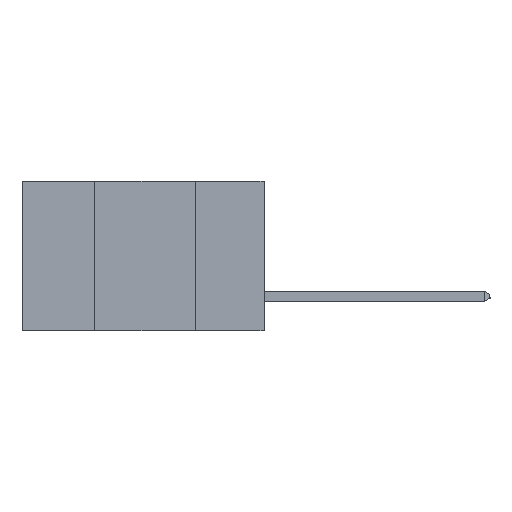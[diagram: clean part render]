
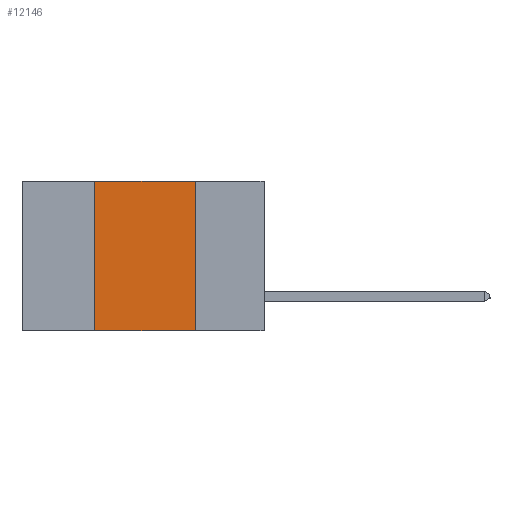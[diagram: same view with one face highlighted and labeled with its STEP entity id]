
A CAD part, left-side view. The second image highlights one B-rep face of the part: STEP entity #12146.
In plain terms, the highlighted planar face has unit normal (-1, 0, 0).
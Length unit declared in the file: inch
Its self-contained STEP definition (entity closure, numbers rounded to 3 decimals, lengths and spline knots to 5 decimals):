
#48 = FACE_OUTER_BOUND ( 'NONE', #1175, .T. ) ;
#1175 = EDGE_LOOP ( 'NONE', ( #3247, #3525, #3396, #16565 ) ) ;
#1203 = PLANE ( 'NONE',  #12071 ) ;
#1386 = VECTOR ( 'NONE', #14968, 39.37008 ) ;
#3179 = LINE ( 'NONE', #13834, #10072 ) ;
#3247 = ORIENTED_EDGE ( 'NONE', *, *, #11730, .F. ) ;
#3396 = ORIENTED_EDGE ( 'NONE', *, *, #7034, .F. ) ;
#3525 = ORIENTED_EDGE ( 'NONE', *, *, #16155, .F. ) ;
#4145 = CARTESIAN_POINT ( 'NONE',  ( 0., 0.42, 0. ) ) ;
#4399 = VECTOR ( 'NONE', #13385, 39.37008 ) ;
#4915 = VERTEX_POINT ( 'NONE', #10560 ) ;
#5005 = LINE ( 'NONE', #8406, #1386 ) ;
#7034 = EDGE_CURVE ( 'NONE', #9112, #10293, #8111, .T. ) ;
#8111 = LINE ( 'NONE', #4145, #4399 ) ;
#8406 = CARTESIAN_POINT ( 'NONE',  ( 0., 0.6, -0.37 ) ) ;
#9112 = VERTEX_POINT ( 'NONE', #11243 ) ;
#9827 = DIRECTION ( 'NONE',  ( 0., 0., -1. ) ) ;
#10072 = VECTOR ( 'NONE', #9827, 39.37008 ) ;
#10293 = VERTEX_POINT ( 'NONE', #15085 ) ;
#10560 = CARTESIAN_POINT ( 'NONE',  ( 0., 0.17, -0.37 ) ) ;
#10762 = DIRECTION ( 'NONE',  ( 0., 0., -1. ) ) ;
#10831 = CARTESIAN_POINT ( 'NONE',  ( 0., 0.6, 0. ) ) ;
#11243 = CARTESIAN_POINT ( 'NONE',  ( 0., 0.42, -0.37 ) ) ;
#11601 = VERTEX_POINT ( 'NONE', #12324 ) ;
#11730 = EDGE_CURVE ( 'NONE', #11601, #4915, #3179, .T. ) ;
#12071 = AXIS2_PLACEMENT_3D ( 'NONE', #17161, #14631, #10762 ) ;
#12146 = ADVANCED_FACE ( 'NONE', ( #48 ), #1203, .F. ) ;
#12324 = CARTESIAN_POINT ( 'NONE',  ( 0., 0.17, 0. ) ) ;
#13385 = DIRECTION ( 'NONE',  ( 0., 0., 1. ) ) ;
#13833 = LINE ( 'NONE', #10831, #17164 ) ;
#13834 = CARTESIAN_POINT ( 'NONE',  ( 0., 0.17, 0. ) ) ;
#14631 = DIRECTION ( 'NONE',  ( 1., 0., 0. ) ) ;
#14968 = DIRECTION ( 'NONE',  ( 0., -1., 0. ) ) ;
#15064 = EDGE_CURVE ( 'NONE', #9112, #4915, #5005, .T. ) ;
#15085 = CARTESIAN_POINT ( 'NONE',  ( 0., 0.42, 0. ) ) ;
#16155 = EDGE_CURVE ( 'NONE', #10293, #11601, #13833, .T. ) ;
#16565 = ORIENTED_EDGE ( 'NONE', *, *, #15064, .T. ) ;
#17161 = CARTESIAN_POINT ( 'NONE',  ( 0., 0.6, 0. ) ) ;
#17164 = VECTOR ( 'NONE', #17223, 39.37008 ) ;
#17223 = DIRECTION ( 'NONE',  ( 0., -1., 0. ) ) ;
